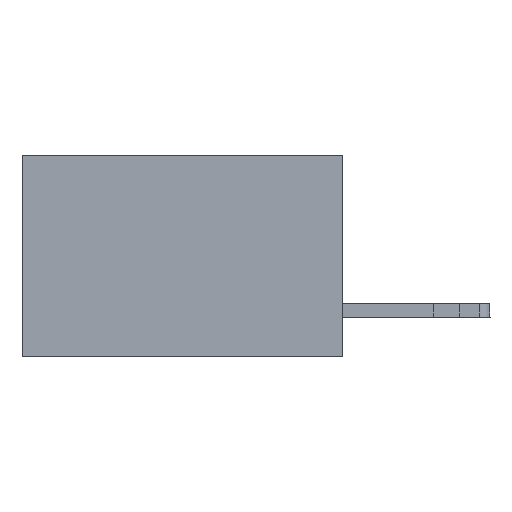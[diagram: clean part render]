
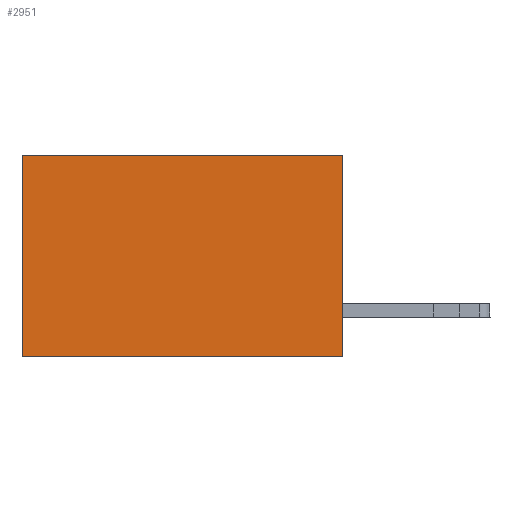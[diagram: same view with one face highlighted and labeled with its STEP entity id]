
A CAD part, left-side view. The second image highlights one B-rep face of the part: STEP entity #2951.
In plain terms, the highlighted planar face has unit normal (-1, 0, 0).
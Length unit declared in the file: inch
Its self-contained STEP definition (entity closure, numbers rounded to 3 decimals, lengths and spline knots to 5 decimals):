
#734 = ORIENTED_EDGE ( 'NONE', *, *, #8495, .F. ) ;
#1208 = AXIS2_PLACEMENT_3D ( 'NONE', #1566, #29108, #28874 ) ;
#1566 = CARTESIAN_POINT ( 'NONE',  ( 0.277, 0., -0.37 ) ) ;
#1623 = PLANE ( 'NONE',  #1208 ) ;
#1634 = FACE_OUTER_BOUND ( 'NONE', #5818, .T. ) ;
#1887 = ORIENTED_EDGE ( 'NONE', *, *, #11092, .F. ) ;
#2951 = ADVANCED_FACE ( 'NONE', ( #1634 ), #1623, .F. ) ;
#3842 = VECTOR ( 'NONE', #24087, 39.37008 ) ;
#5368 = LINE ( 'NONE', #9439, #30361 ) ;
#5818 = EDGE_LOOP ( 'NONE', ( #17568, #1887, #734, #29808 ) ) ;
#6494 = VERTEX_POINT ( 'NONE', #14654 ) ;
#7218 = VERTEX_POINT ( 'NONE', #19520 ) ;
#8495 = EDGE_CURVE ( 'NONE', #7218, #20751, #28613, .T. ) ;
#9408 = DIRECTION ( 'NONE',  ( 0., 0., -1. ) ) ;
#9439 = CARTESIAN_POINT ( 'NONE',  ( 0.277, 0.59, -0.37 ) ) ;
#11092 = EDGE_CURVE ( 'NONE', #20751, #6494, #16766, .T. ) ;
#11534 = EDGE_CURVE ( 'NONE', #7218, #30027, #22110, .T. ) ;
#12070 = EDGE_CURVE ( 'NONE', #30027, #6494, #5368, .T. ) ;
#13294 = CARTESIAN_POINT ( 'NONE',  ( 0.277, 0.59, 0. ) ) ;
#14654 = CARTESIAN_POINT ( 'NONE',  ( 0.277, 0.59, -0.37 ) ) ;
#15633 = VECTOR ( 'NONE', #17524, 39.37008 ) ;
#16766 = LINE ( 'NONE', #24252, #3842 ) ;
#17266 = CARTESIAN_POINT ( 'NONE',  ( 0.277, 0., -0.37 ) ) ;
#17524 = DIRECTION ( 'NONE',  ( 0., 1., 0. ) ) ;
#17568 = ORIENTED_EDGE ( 'NONE', *, *, #12070, .T. ) ;
#17737 = CARTESIAN_POINT ( 'NONE',  ( 0.277, 0., 0. ) ) ;
#19316 = CARTESIAN_POINT ( 'NONE',  ( 0.277, 0., -0.37 ) ) ;
#19324 = DIRECTION ( 'NONE',  ( 0., 0., -1. ) ) ;
#19520 = CARTESIAN_POINT ( 'NONE',  ( 0.277, 0., 0. ) ) ;
#20751 = VERTEX_POINT ( 'NONE', #17266 ) ;
#22110 = LINE ( 'NONE', #17737, #15633 ) ;
#24087 = DIRECTION ( 'NONE',  ( 0., 1., 0. ) ) ;
#24252 = CARTESIAN_POINT ( 'NONE',  ( 0.277, 0., -0.37 ) ) ;
#28613 = LINE ( 'NONE', #19316, #29360 ) ;
#28874 = DIRECTION ( 'NONE',  ( 0., 0., -1. ) ) ;
#29108 = DIRECTION ( 'NONE',  ( 1., 0., 0. ) ) ;
#29360 = VECTOR ( 'NONE', #19324, 39.37008 ) ;
#29808 = ORIENTED_EDGE ( 'NONE', *, *, #11534, .T. ) ;
#30027 = VERTEX_POINT ( 'NONE', #13294 ) ;
#30361 = VECTOR ( 'NONE', #9408, 39.37008 ) ;
